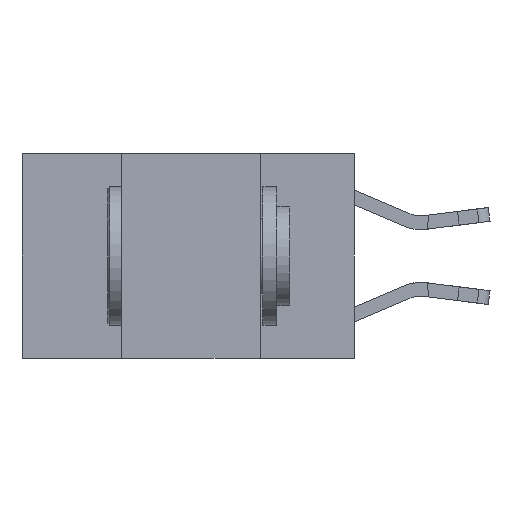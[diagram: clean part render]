
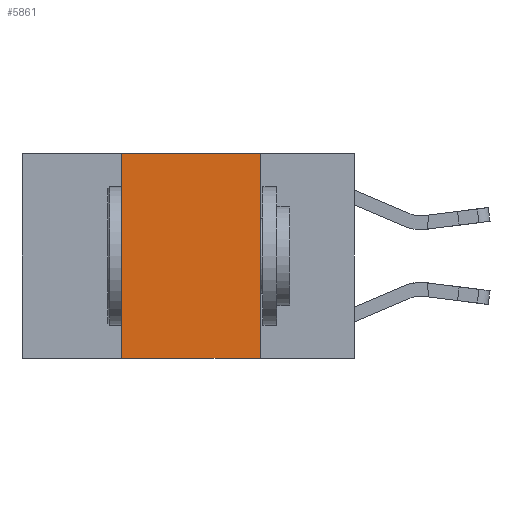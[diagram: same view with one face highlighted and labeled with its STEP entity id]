
A CAD part, left-side view. The second image highlights one B-rep face of the part: STEP entity #5861.
In plain terms, the highlighted planar face has unit normal (-1, 0, 0).
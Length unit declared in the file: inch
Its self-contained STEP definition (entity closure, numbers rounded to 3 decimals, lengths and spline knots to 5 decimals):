
#165 = CARTESIAN_POINT ( 'NONE',  ( 0., 0.42, -0.37 ) ) ;
#1349 = DIRECTION ( 'NONE',  ( 0., 0., 1. ) ) ;
#1465 = CARTESIAN_POINT ( 'NONE',  ( 0., 0.42, 0. ) ) ;
#2732 = DIRECTION ( 'NONE',  ( 1., 0., 0. ) ) ;
#3312 = ORIENTED_EDGE ( 'NONE', *, *, #13815, .F. ) ;
#4250 = DIRECTION ( 'NONE',  ( 0., 0., -1. ) ) ;
#4946 = ORIENTED_EDGE ( 'NONE', *, *, #19414, .T. ) ;
#4993 = EDGE_CURVE ( 'NONE', #17158, #17013, #18294, .T. ) ;
#5684 = DIRECTION ( 'NONE',  ( 0., -1., 0. ) ) ;
#5861 = ADVANCED_FACE ( 'NONE', ( #18159 ), #16727, .F. ) ;
#7472 = ORIENTED_EDGE ( 'NONE', *, *, #18376, .F. ) ;
#8419 = VECTOR ( 'NONE', #4250, 39.37008 ) ;
#8682 = CARTESIAN_POINT ( 'NONE',  ( 0., 0.6, 0. ) ) ;
#9201 = VECTOR ( 'NONE', #18491, 39.37008 ) ;
#9373 = EDGE_LOOP ( 'NONE', ( #3312, #7472, #18141, #4946 ) ) ;
#9512 = VECTOR ( 'NONE', #5684, 39.37008 ) ;
#10445 = CARTESIAN_POINT ( 'NONE',  ( 0., 0.17, 0. ) ) ;
#11853 = DIRECTION ( 'NONE',  ( 0., 0., -1. ) ) ;
#11869 = CARTESIAN_POINT ( 'NONE',  ( 0., 0.42, 0. ) ) ;
#12247 = AXIS2_PLACEMENT_3D ( 'NONE', #8682, #2732, #11853 ) ;
#12437 = VERTEX_POINT ( 'NONE', #19876 ) ;
#13815 = EDGE_CURVE ( 'NONE', #19402, #12437, #18554, .T. ) ;
#15358 = LINE ( 'NONE', #18388, #9201 ) ;
#16417 = LINE ( 'NONE', #17931, #9512 ) ;
#16446 = VECTOR ( 'NONE', #1349, 39.37008 ) ;
#16727 = PLANE ( 'NONE',  #12247 ) ;
#17013 = VERTEX_POINT ( 'NONE', #11869 ) ;
#17158 = VERTEX_POINT ( 'NONE', #165 ) ;
#17931 = CARTESIAN_POINT ( 'NONE',  ( 0., 0.6, 0. ) ) ;
#18141 = ORIENTED_EDGE ( 'NONE', *, *, #4993, .F. ) ;
#18159 = FACE_OUTER_BOUND ( 'NONE', #9373, .T. ) ;
#18294 = LINE ( 'NONE', #1465, #16446 ) ;
#18376 = EDGE_CURVE ( 'NONE', #17013, #19402, #16417, .T. ) ;
#18388 = CARTESIAN_POINT ( 'NONE',  ( 0., 0.6, -0.37 ) ) ;
#18466 = CARTESIAN_POINT ( 'NONE',  ( 0., 0.17, 0. ) ) ;
#18491 = DIRECTION ( 'NONE',  ( 0., -1., 0. ) ) ;
#18554 = LINE ( 'NONE', #18466, #8419 ) ;
#19402 = VERTEX_POINT ( 'NONE', #10445 ) ;
#19414 = EDGE_CURVE ( 'NONE', #17158, #12437, #15358, .T. ) ;
#19876 = CARTESIAN_POINT ( 'NONE',  ( 0., 0.17, -0.37 ) ) ;
